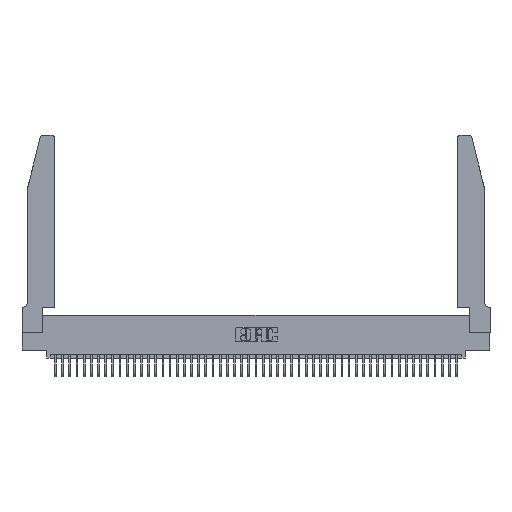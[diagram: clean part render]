
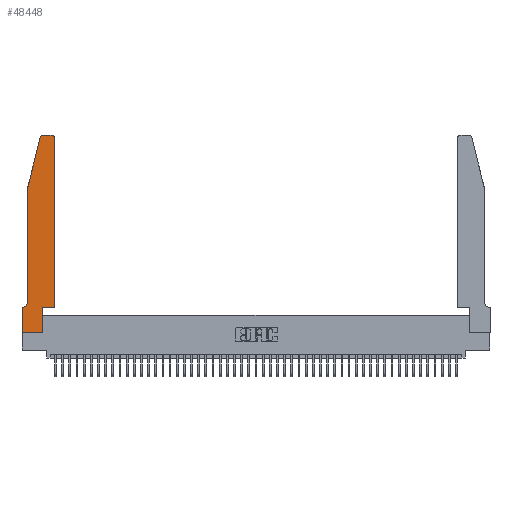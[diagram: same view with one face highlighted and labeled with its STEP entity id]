
A CAD part, top view. The second image highlights one B-rep face of the part: STEP entity #48448.
In plain terms, the highlighted planar face has unit normal (0, 0, 1).
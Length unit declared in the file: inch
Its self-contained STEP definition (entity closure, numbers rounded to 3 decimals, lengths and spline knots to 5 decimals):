
#1522 = ORIENTED_EDGE ( 'NONE', *, *, #18503, .T. ) ;
#1663 = DIRECTION ( 'NONE',  ( 1., 0., 0. ) ) ;
#1869 = CARTESIAN_POINT ( 'NONE',  ( 0., 0., 0.37 ) ) ;
#2078 = EDGE_CURVE ( 'NONE', #15184, #41891, #4046, .T. ) ;
#3019 = CARTESIAN_POINT ( 'NONE',  ( 0.0755, 2., 0.37 ) ) ;
#3157 = VECTOR ( 'NONE', #38509, 39.37008 ) ;
#3288 = DIRECTION ( 'NONE',  ( 1., 0., 0. ) ) ;
#4046 = CIRCLE ( 'NONE', #11628, 0.03 ) ;
#4095 = VERTEX_POINT ( 'NONE', #27155 ) ;
#4183 = DIRECTION ( 'NONE',  ( 0., 0., 1. ) ) ;
#4975 = VERTEX_POINT ( 'NONE', #36042 ) ;
#5234 = CARTESIAN_POINT ( 'NONE',  ( 0.4505, 2.72, 0.37 ) ) ;
#5335 = EDGE_CURVE ( 'NONE', #32245, #10756, #37177, .T. ) ;
#6950 = EDGE_CURVE ( 'NONE', #34010, #11494, #28652, .T. ) ;
#7411 = AXIS2_PLACEMENT_3D ( 'NONE', #39693, #16924, #43484 ) ;
#7913 = LINE ( 'NONE', #17640, #44785 ) ;
#8064 = CARTESIAN_POINT ( 'NONE',  ( 0.0755, 0.35, 0.37 ) ) ;
#8484 = VECTOR ( 'NONE', #1663, 39.37008 ) ;
#8575 = VERTEX_POINT ( 'NONE', #25229 ) ;
#8588 = ORIENTED_EDGE ( 'NONE', *, *, #38721, .T. ) ;
#8644 = ORIENTED_EDGE ( 'NONE', *, *, #18504, .T. ) ;
#8836 = CARTESIAN_POINT ( 'NONE',  ( 0., 0.35, 0.37 ) ) ;
#10016 = LINE ( 'NONE', #1869, #40404 ) ;
#10756 = VERTEX_POINT ( 'NONE', #28710 ) ;
#10998 = AXIS2_PLACEMENT_3D ( 'NONE', #8836, #43073, #20343 ) ;
#11384 = CARTESIAN_POINT ( 'NONE',  ( 0.0755, 2., 0.37 ) ) ;
#11494 = VERTEX_POINT ( 'NONE', #13946 ) ;
#11628 = AXIS2_PLACEMENT_3D ( 'NONE', #48851, #26143, #3288 ) ;
#12146 = ORIENTED_EDGE ( 'NONE', *, *, #2078, .T. ) ;
#12883 = VERTEX_POINT ( 'NONE', #33723 ) ;
#13611 = ORIENTED_EDGE ( 'NONE', *, *, #17648, .T. ) ;
#13946 = CARTESIAN_POINT ( 'NONE',  ( 0.25487, 2.72718, 0.37 ) ) ;
#14490 = DIRECTION ( 'NONE',  ( -0.239, -0.971, 0. ) ) ;
#15138 = LINE ( 'NONE', #24445, #34216 ) ;
#15184 = VERTEX_POINT ( 'NONE', #5234 ) ;
#15199 = CARTESIAN_POINT ( 'NONE',  ( 0.0755, 2., 0.37 ) ) ;
#16484 = ORIENTED_EDGE ( 'NONE', *, *, #35452, .T. ) ;
#16523 = PLANE ( 'NONE',  #10998 ) ;
#16924 = DIRECTION ( 'NONE',  ( 0., 0., -1. ) ) ;
#16936 = VECTOR ( 'NONE', #19039, 39.37008 ) ;
#17640 = CARTESIAN_POINT ( 'NONE',  ( 0.4505, 0.35, 0.37 ) ) ;
#17648 = EDGE_CURVE ( 'NONE', #10756, #4095, #22294, .T. ) ;
#17806 = DIRECTION ( 'NONE',  ( 0., 1., 0. ) ) ;
#18390 = ORIENTED_EDGE ( 'NONE', *, *, #37395, .T. ) ;
#18503 = EDGE_CURVE ( 'NONE', #47425, #20991, #28178, .T. ) ;
#18504 = EDGE_CURVE ( 'NONE', #4975, #15184, #7913, .T. ) ;
#19039 = DIRECTION ( 'NONE',  ( 0., -1., 0. ) ) ;
#19130 = LINE ( 'NONE', #23665, #38169 ) ;
#20343 = DIRECTION ( 'NONE',  ( 1., 0., 0. ) ) ;
#20598 = DIRECTION ( 'NONE',  ( -1., 0., 0. ) ) ;
#20725 = CARTESIAN_POINT ( 'NONE',  ( 0.284, 2.75, 0.37 ) ) ;
#20991 = VERTEX_POINT ( 'NONE', #21080 ) ;
#21014 = FACE_OUTER_BOUND ( 'NONE', #45150, .T. ) ;
#21080 = CARTESIAN_POINT ( 'NONE',  ( 0.2865, 0.35, 0.37 ) ) ;
#21618 = DIRECTION ( 'NONE',  ( 0., 1., 0. ) ) ;
#21714 = ORIENTED_EDGE ( 'NONE', *, *, #27013, .T. ) ;
#22294 = CIRCLE ( 'NONE', #7411, 0.07 ) ;
#23665 = CARTESIAN_POINT ( 'NONE',  ( 0., 0., 0.37 ) ) ;
#24445 = CARTESIAN_POINT ( 'NONE',  ( 0.2605, 2.75, 0.37 ) ) ;
#24508 = CARTESIAN_POINT ( 'NONE',  ( 0.4505, 0.35, 0.37 ) ) ;
#24709 = DIRECTION ( 'NONE',  ( 0., -1., 0. ) ) ;
#25229 = CARTESIAN_POINT ( 'NONE',  ( 0., 0.35, 0.37 ) ) ;
#25258 = CARTESIAN_POINT ( 'NONE',  ( 0.2865, 0., 0.37 ) ) ;
#26143 = DIRECTION ( 'NONE',  ( 0., 0., 1. ) ) ;
#27013 = EDGE_CURVE ( 'NONE', #4095, #8575, #32361, .T. ) ;
#27036 = CARTESIAN_POINT ( 'NONE',  ( 0.284, 2.72, 0.37 ) ) ;
#27126 = CARTESIAN_POINT ( 'NONE',  ( 0.4205, 2.75, 0.37 ) ) ;
#27155 = CARTESIAN_POINT ( 'NONE',  ( 0.0055, 0.35, 0.37 ) ) ;
#27505 = DIRECTION ( 'NONE',  ( 1., 0., 0. ) ) ;
#27792 = VECTOR ( 'NONE', #14490, 39.37008 ) ;
#28178 = LINE ( 'NONE', #40572, #35912 ) ;
#28652 = CIRCLE ( 'NONE', #36695, 0.03 ) ;
#28710 = CARTESIAN_POINT ( 'NONE',  ( 0.0755, 0.42, 0.37 ) ) ;
#29616 = ORIENTED_EDGE ( 'NONE', *, *, #5335, .T. ) ;
#30874 = DIRECTION ( 'NONE',  ( 1., 0., 0. ) ) ;
#31008 = EDGE_CURVE ( 'NONE', #11494, #32245, #37900, .T. ) ;
#32245 = VERTEX_POINT ( 'NONE', #11384 ) ;
#32361 = LINE ( 'NONE', #8064, #3157 ) ;
#33723 = CARTESIAN_POINT ( 'NONE',  ( 0., 0., 0.37 ) ) ;
#34010 = VERTEX_POINT ( 'NONE', #20725 ) ;
#34216 = VECTOR ( 'NONE', #20598, 39.37008 ) ;
#35452 = EDGE_CURVE ( 'NONE', #41891, #34010, #15138, .T. ) ;
#35912 = VECTOR ( 'NONE', #17806, 39.37008 ) ;
#36042 = CARTESIAN_POINT ( 'NONE',  ( 0.4505, 0.35, 0.37 ) ) ;
#36695 = AXIS2_PLACEMENT_3D ( 'NONE', #27036, #4183, #30874 ) ;
#37177 = LINE ( 'NONE', #15199, #16936 ) ;
#37395 = EDGE_CURVE ( 'NONE', #12883, #47425, #19130, .T. ) ;
#37900 = LINE ( 'NONE', #3019, #27792 ) ;
#38169 = VECTOR ( 'NONE', #27505, 39.37008 ) ;
#38509 = DIRECTION ( 'NONE',  ( -1., 0., 0. ) ) ;
#38721 = EDGE_CURVE ( 'NONE', #8575, #12883, #10016, .T. ) ;
#39693 = CARTESIAN_POINT ( 'NONE',  ( 0.0055, 0.42, 0.37 ) ) ;
#40404 = VECTOR ( 'NONE', #24709, 39.37008 ) ;
#40572 = CARTESIAN_POINT ( 'NONE',  ( 0.2865, 0.35, 0.37 ) ) ;
#41891 = VERTEX_POINT ( 'NONE', #27126 ) ;
#43073 = DIRECTION ( 'NONE',  ( 0., 0., 1. ) ) ;
#43484 = DIRECTION ( 'NONE',  ( -1., 0., 0. ) ) ;
#44642 = ORIENTED_EDGE ( 'NONE', *, *, #6950, .T. ) ;
#44785 = VECTOR ( 'NONE', #21618, 39.37008 ) ;
#45150 = EDGE_LOOP ( 'NONE', ( #16484, #44642, #46465, #29616, #13611, #21714, #8588, #18390, #1522, #47694, #8644, #12146 ) ) ;
#46465 = ORIENTED_EDGE ( 'NONE', *, *, #31008, .T. ) ;
#47425 = VERTEX_POINT ( 'NONE', #25258 ) ;
#47694 = ORIENTED_EDGE ( 'NONE', *, *, #48517, .T. ) ;
#48448 = ADVANCED_FACE ( 'NONE', ( #21014 ), #16523, .T. ) ;
#48517 = EDGE_CURVE ( 'NONE', #20991, #4975, #48931, .T. ) ;
#48851 = CARTESIAN_POINT ( 'NONE',  ( 0.4205, 2.72, 0.37 ) ) ;
#48931 = LINE ( 'NONE', #24508, #8484 ) ;
